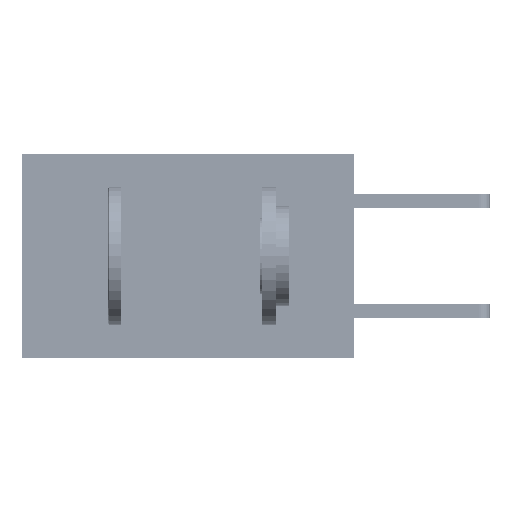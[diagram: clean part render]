
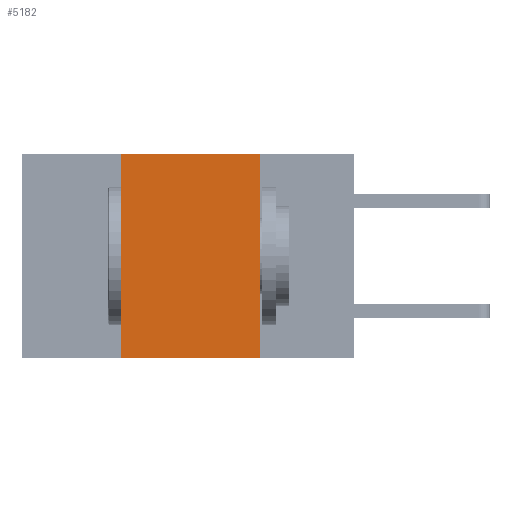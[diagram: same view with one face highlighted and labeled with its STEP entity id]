
A CAD part, left-side view. The second image highlights one B-rep face of the part: STEP entity #5182.
In plain terms, the highlighted planar face has unit normal (-1, 0, 0).
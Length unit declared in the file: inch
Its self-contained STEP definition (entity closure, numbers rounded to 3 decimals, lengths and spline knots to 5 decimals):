
#1597 = VERTEX_POINT ( 'NONE', #9426 ) ;
#4119 = DIRECTION ( 'NONE',  ( 0., 0., 1. ) ) ;
#5045 = VERTEX_POINT ( 'NONE', #15741 ) ;
#5182 = ADVANCED_FACE ( 'NONE', ( #43031 ), #19720, .F. ) ;
#6180 = CARTESIAN_POINT ( 'NONE',  ( 0., 0.17, 0. ) ) ;
#7040 = ORIENTED_EDGE ( 'NONE', *, *, #19374, .F. ) ;
#9426 = CARTESIAN_POINT ( 'NONE',  ( 0., 0.17, -0.37 ) ) ;
#10081 = VECTOR ( 'NONE', #32100, 39.37008 ) ;
#11796 = ORIENTED_EDGE ( 'NONE', *, *, #22511, .T. ) ;
#12102 = CARTESIAN_POINT ( 'NONE',  ( 0., 0.17, 0. ) ) ;
#14289 = CARTESIAN_POINT ( 'NONE',  ( 0., 0.42, 0. ) ) ;
#15341 = VECTOR ( 'NONE', #28177, 39.37008 ) ;
#15741 = CARTESIAN_POINT ( 'NONE',  ( 0., 0.42, -0.37 ) ) ;
#16546 = LINE ( 'NONE', #21233, #24424 ) ;
#18782 = ORIENTED_EDGE ( 'NONE', *, *, #23708, .F. ) ;
#19374 = EDGE_CURVE ( 'NONE', #5045, #22717, #25279, .T. ) ;
#19426 = DIRECTION ( 'NONE',  ( 0., 0., -1. ) ) ;
#19720 = PLANE ( 'NONE',  #30472 ) ;
#20039 = EDGE_CURVE ( 'NONE', #22717, #38549, #30583, .T. ) ;
#21233 = CARTESIAN_POINT ( 'NONE',  ( 0., 0.6, -0.37 ) ) ;
#21807 = ORIENTED_EDGE ( 'NONE', *, *, #20039, .F. ) ;
#22511 = EDGE_CURVE ( 'NONE', #5045, #1597, #16546, .T. ) ;
#22717 = VERTEX_POINT ( 'NONE', #14289 ) ;
#23091 = DIRECTION ( 'NONE',  ( 1., 0., 0. ) ) ;
#23708 = EDGE_CURVE ( 'NONE', #38549, #1597, #29064, .T. ) ;
#24139 = CARTESIAN_POINT ( 'NONE',  ( 0., 0.42, 0. ) ) ;
#24424 = VECTOR ( 'NONE', #34247, 39.37008 ) ;
#25279 = LINE ( 'NONE', #24139, #26324 ) ;
#26324 = VECTOR ( 'NONE', #4119, 39.37008 ) ;
#26605 = CARTESIAN_POINT ( 'NONE',  ( 0., 0.6, 0. ) ) ;
#28177 = DIRECTION ( 'NONE',  ( 0., -1., 0. ) ) ;
#29064 = LINE ( 'NONE', #12102, #10081 ) ;
#30472 = AXIS2_PLACEMENT_3D ( 'NONE', #26605, #23091, #19426 ) ;
#30583 = LINE ( 'NONE', #41466, #15341 ) ;
#32100 = DIRECTION ( 'NONE',  ( 0., 0., -1. ) ) ;
#34247 = DIRECTION ( 'NONE',  ( 0., -1., 0. ) ) ;
#38549 = VERTEX_POINT ( 'NONE', #6180 ) ;
#38688 = EDGE_LOOP ( 'NONE', ( #18782, #21807, #7040, #11796 ) ) ;
#41466 = CARTESIAN_POINT ( 'NONE',  ( 0., 0.6, 0. ) ) ;
#43031 = FACE_OUTER_BOUND ( 'NONE', #38688, .T. ) ;
